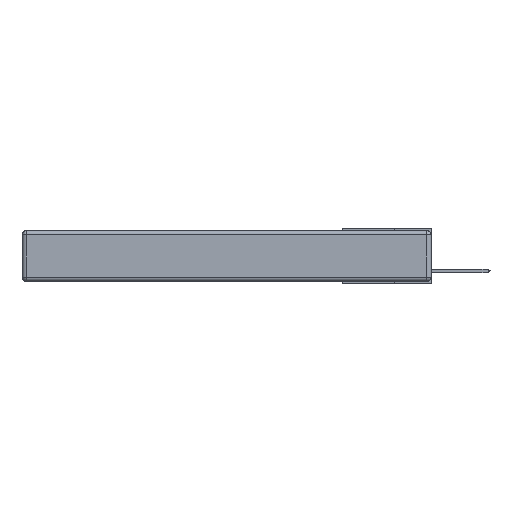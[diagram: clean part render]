
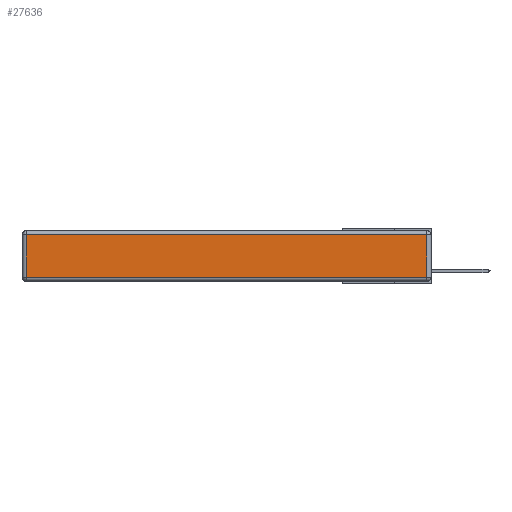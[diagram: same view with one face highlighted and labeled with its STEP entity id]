
A CAD part, left-side view. The second image highlights one B-rep face of the part: STEP entity #27636.
In plain terms, the highlighted planar face has unit normal (-1, 0, 0).
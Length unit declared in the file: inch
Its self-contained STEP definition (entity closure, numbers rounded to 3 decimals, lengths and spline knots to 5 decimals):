
#141 = VERTEX_POINT ( 'NONE', #25432 ) ;
#749 = EDGE_CURVE ( 'NONE', #8834, #141, #6549, .T. ) ;
#1113 = CARTESIAN_POINT ( 'NONE',  ( 0., 0.03, -0.03 ) ) ;
#1858 = ORIENTED_EDGE ( 'NONE', *, *, #749, .T. ) ;
#2158 = VERTEX_POINT ( 'NONE', #26834 ) ;
#3149 = ORIENTED_EDGE ( 'NONE', *, *, #11788, .T. ) ;
#5086 = CARTESIAN_POINT ( 'NONE',  ( 0., 2.75, -0.03 ) ) ;
#5213 = CARTESIAN_POINT ( 'NONE',  ( 0., 2.72, -0.313 ) ) ;
#5902 = DIRECTION ( 'NONE',  ( 0., -1., 0. ) ) ;
#6549 = LINE ( 'NONE', #17362, #29223 ) ;
#7913 = ORIENTED_EDGE ( 'NONE', *, *, #21279, .T. ) ;
#8304 = LINE ( 'NONE', #25828, #21822 ) ;
#8834 = VERTEX_POINT ( 'NONE', #5213 ) ;
#11503 = EDGE_CURVE ( 'NONE', #2158, #8834, #8304, .T. ) ;
#11788 = EDGE_CURVE ( 'NONE', #141, #27231, #17056, .T. ) ;
#12252 = FACE_OUTER_BOUND ( 'NONE', #17242, .T. ) ;
#14125 = PLANE ( 'NONE',  #30178 ) ;
#16757 = VECTOR ( 'NONE', #28617, 39.37008 ) ;
#17056 = LINE ( 'NONE', #17060, #25503 ) ;
#17060 = CARTESIAN_POINT ( 'NONE',  ( 0., 0.03, -0.343 ) ) ;
#17097 = LINE ( 'NONE', #5086, #16757 ) ;
#17242 = EDGE_LOOP ( 'NONE', ( #1858, #3149, #7913, #27940 ) ) ;
#17362 = CARTESIAN_POINT ( 'NONE',  ( 0., 0., -0.313 ) ) ;
#19033 = DIRECTION ( 'NONE',  ( 0., 0., -1. ) ) ;
#20883 = DIRECTION ( 'NONE',  ( 0., 0., 1. ) ) ;
#21279 = EDGE_CURVE ( 'NONE', #27231, #2158, #17097, .T. ) ;
#21822 = VECTOR ( 'NONE', #19033, 39.37008 ) ;
#23337 = DIRECTION ( 'NONE',  ( -1., 0., 0. ) ) ;
#25432 = CARTESIAN_POINT ( 'NONE',  ( 0., 0.03, -0.313 ) ) ;
#25503 = VECTOR ( 'NONE', #28327, 39.37008 ) ;
#25828 = CARTESIAN_POINT ( 'NONE',  ( 0., 2.72, -0.343 ) ) ;
#26834 = CARTESIAN_POINT ( 'NONE',  ( 0., 2.72, -0.03 ) ) ;
#27231 = VERTEX_POINT ( 'NONE', #1113 ) ;
#27636 = ADVANCED_FACE ( 'NONE', ( #12252 ), #14125, .T. ) ;
#27940 = ORIENTED_EDGE ( 'NONE', *, *, #11503, .T. ) ;
#27953 = CARTESIAN_POINT ( 'NONE',  ( 0., 0., -0.343 ) ) ;
#28327 = DIRECTION ( 'NONE',  ( 0., 0., 1. ) ) ;
#28617 = DIRECTION ( 'NONE',  ( 0., 1., 0. ) ) ;
#29223 = VECTOR ( 'NONE', #5902, 39.37008 ) ;
#30178 = AXIS2_PLACEMENT_3D ( 'NONE', #27953, #23337, #20883 ) ;
